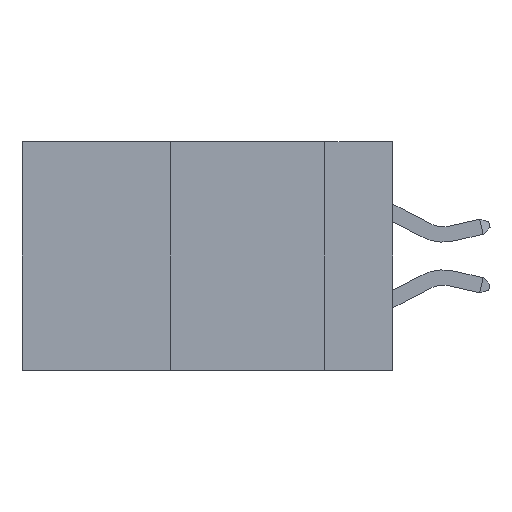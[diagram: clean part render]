
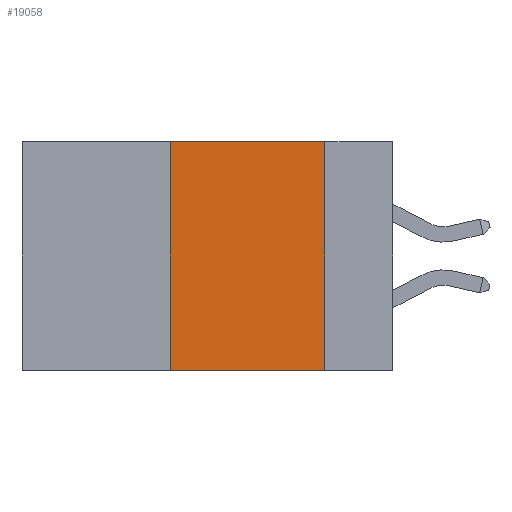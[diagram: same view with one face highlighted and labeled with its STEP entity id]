
A CAD part, left-side view. The second image highlights one B-rep face of the part: STEP entity #19058.
In plain terms, the highlighted planar face has unit normal (-1, 0, 0).
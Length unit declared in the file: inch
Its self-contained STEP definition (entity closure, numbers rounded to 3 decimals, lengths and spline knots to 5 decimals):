
#3733 = LINE ( 'NONE', #33703, #32362 ) ;
#3787 = CARTESIAN_POINT ( 'NONE',  ( 0., 0.11, 0. ) ) ;
#3825 = CARTESIAN_POINT ( 'NONE',  ( 0., 0.36, 0. ) ) ;
#3895 = DIRECTION ( 'NONE',  ( 0., -1., 0. ) ) ;
#4704 = EDGE_CURVE ( 'NONE', #41891, #8368, #24963, .T. ) ;
#8368 = VERTEX_POINT ( 'NONE', #22624 ) ;
#11917 = AXIS2_PLACEMENT_3D ( 'NONE', #14238, #35169, #24326 ) ;
#14238 = CARTESIAN_POINT ( 'NONE',  ( 0., 0.6, 0. ) ) ;
#14455 = EDGE_CURVE ( 'NONE', #8368, #27853, #33772, .T. ) ;
#15042 = EDGE_LOOP ( 'NONE', ( #38750, #30468, #21684, #25839 ) ) ;
#16670 = VECTOR ( 'NONE', #3895, 39.37008 ) ;
#17326 = CARTESIAN_POINT ( 'NONE',  ( 0., 0.6, 0. ) ) ;
#17491 = VERTEX_POINT ( 'NONE', #35740 ) ;
#19058 = ADVANCED_FACE ( 'NONE', ( #21044 ), #37805, .F. ) ;
#21044 = FACE_OUTER_BOUND ( 'NONE', #15042, .T. ) ;
#21452 = EDGE_CURVE ( 'NONE', #17491, #27853, #3733, .T. ) ;
#21684 = ORIENTED_EDGE ( 'NONE', *, *, #28377, .F. ) ;
#21769 = VECTOR ( 'NONE', #23864, 39.37008 ) ;
#22624 = CARTESIAN_POINT ( 'NONE',  ( 0., 0.11, 0. ) ) ;
#23864 = DIRECTION ( 'NONE',  ( 0., 0., 1. ) ) ;
#24326 = DIRECTION ( 'NONE',  ( 0., 0., -1. ) ) ;
#24963 = LINE ( 'NONE', #17326, #16670 ) ;
#25839 = ORIENTED_EDGE ( 'NONE', *, *, #21452, .T. ) ;
#27853 = VERTEX_POINT ( 'NONE', #33228 ) ;
#28377 = EDGE_CURVE ( 'NONE', #17491, #41891, #36701, .T. ) ;
#29932 = DIRECTION ( 'NONE',  ( 0., -1., 0. ) ) ;
#30468 = ORIENTED_EDGE ( 'NONE', *, *, #4704, .F. ) ;
#32362 = VECTOR ( 'NONE', #29932, 39.37008 ) ;
#33228 = CARTESIAN_POINT ( 'NONE',  ( 0., 0.11, -0.37 ) ) ;
#33703 = CARTESIAN_POINT ( 'NONE',  ( 0., 0.6, -0.37 ) ) ;
#33772 = LINE ( 'NONE', #3787, #33898 ) ;
#33898 = VECTOR ( 'NONE', #34199, 39.37008 ) ;
#34199 = DIRECTION ( 'NONE',  ( 0., 0., -1. ) ) ;
#35169 = DIRECTION ( 'NONE',  ( 1., 0., 0. ) ) ;
#35740 = CARTESIAN_POINT ( 'NONE',  ( 0., 0.36, -0.37 ) ) ;
#35771 = CARTESIAN_POINT ( 'NONE',  ( 0., 0.36, 0. ) ) ;
#36701 = LINE ( 'NONE', #3825, #21769 ) ;
#37805 = PLANE ( 'NONE',  #11917 ) ;
#38750 = ORIENTED_EDGE ( 'NONE', *, *, #14455, .F. ) ;
#41891 = VERTEX_POINT ( 'NONE', #35771 ) ;
